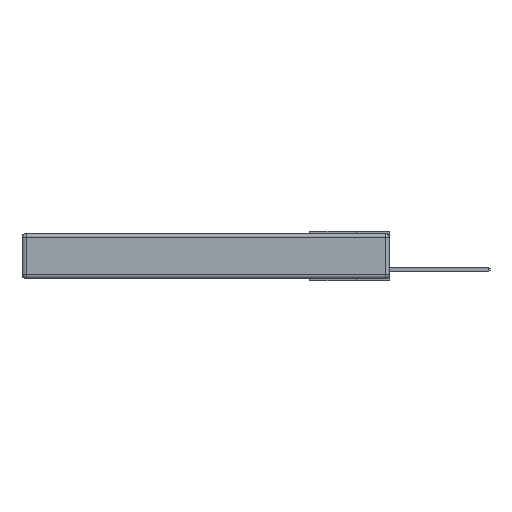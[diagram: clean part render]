
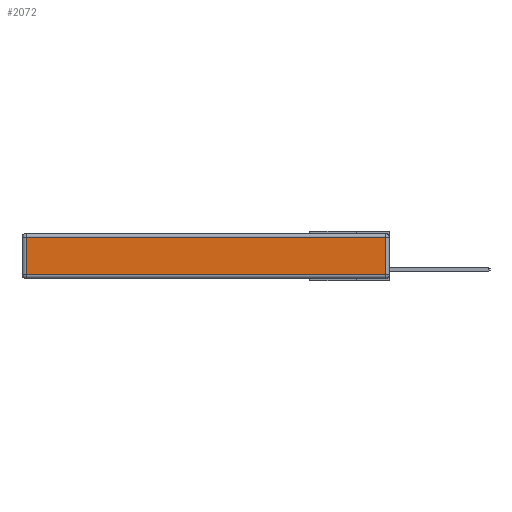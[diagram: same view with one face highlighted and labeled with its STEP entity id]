
A CAD part, left-side view. The second image highlights one B-rep face of the part: STEP entity #2072.
In plain terms, the highlighted planar face has unit normal (-1, 0, 0).
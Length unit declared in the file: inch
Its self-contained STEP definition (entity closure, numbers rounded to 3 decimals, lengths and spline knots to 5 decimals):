
#176 = CARTESIAN_POINT ( 'NONE',  ( 0., 0.03, -0.03 ) ) ;
#444 = VECTOR ( 'NONE', #2359, 39.37008 ) ;
#1381 = CARTESIAN_POINT ( 'NONE',  ( 0., 0.03, -0.313 ) ) ;
#2072 = ADVANCED_FACE ( 'NONE', ( #6727 ), #2088, .T. ) ;
#2088 = PLANE ( 'NONE',  #13191 ) ;
#2359 = DIRECTION ( 'NONE',  ( 0., 1., 0. ) ) ;
#3408 = VERTEX_POINT ( 'NONE', #4120 ) ;
#4120 = CARTESIAN_POINT ( 'NONE',  ( 0., 2.72, -0.313 ) ) ;
#4215 = DIRECTION ( 'NONE',  ( 0., 0., 1. ) ) ;
#4697 = LINE ( 'NONE', #11352, #8813 ) ;
#4736 = DIRECTION ( 'NONE',  ( 0., 0., 1. ) ) ;
#5076 = DIRECTION ( 'NONE',  ( 0., 0., -1. ) ) ;
#5177 = CARTESIAN_POINT ( 'NONE',  ( 0., 2.72, -0.03 ) ) ;
#5484 = CARTESIAN_POINT ( 'NONE',  ( 0., 0.03, -0.343 ) ) ;
#5848 = EDGE_CURVE ( 'NONE', #9457, #11286, #15091, .T. ) ;
#5866 = DIRECTION ( 'NONE',  ( 0., -1., 0. ) ) ;
#6336 = CARTESIAN_POINT ( 'NONE',  ( 0., 2.75, -0.03 ) ) ;
#6727 = FACE_OUTER_BOUND ( 'NONE', #15575, .T. ) ;
#7026 = ORIENTED_EDGE ( 'NONE', *, *, #15288, .T. ) ;
#8813 = VECTOR ( 'NONE', #5866, 39.37008 ) ;
#9131 = ORIENTED_EDGE ( 'NONE', *, *, #14897, .T. ) ;
#9163 = ORIENTED_EDGE ( 'NONE', *, *, #5848, .T. ) ;
#9457 = VERTEX_POINT ( 'NONE', #176 ) ;
#9525 = VERTEX_POINT ( 'NONE', #1381 ) ;
#10279 = CARTESIAN_POINT ( 'NONE',  ( 0., 0., -0.343 ) ) ;
#11286 = VERTEX_POINT ( 'NONE', #5177 ) ;
#11352 = CARTESIAN_POINT ( 'NONE',  ( 0., 0., -0.313 ) ) ;
#11611 = DIRECTION ( 'NONE',  ( -1., 0., 0. ) ) ;
#12475 = VECTOR ( 'NONE', #5076, 39.37008 ) ;
#12893 = VECTOR ( 'NONE', #4215, 39.37008 ) ;
#13191 = AXIS2_PLACEMENT_3D ( 'NONE', #10279, #11611, #4736 ) ;
#14405 = LINE ( 'NONE', #17434, #12475 ) ;
#14701 = EDGE_CURVE ( 'NONE', #11286, #3408, #14405, .T. ) ;
#14812 = ORIENTED_EDGE ( 'NONE', *, *, #14701, .T. ) ;
#14897 = EDGE_CURVE ( 'NONE', #3408, #9525, #4697, .T. ) ;
#15091 = LINE ( 'NONE', #6336, #444 ) ;
#15288 = EDGE_CURVE ( 'NONE', #9525, #9457, #16995, .T. ) ;
#15575 = EDGE_LOOP ( 'NONE', ( #9131, #7026, #9163, #14812 ) ) ;
#16995 = LINE ( 'NONE', #5484, #12893 ) ;
#17434 = CARTESIAN_POINT ( 'NONE',  ( 0., 2.72, -0.343 ) ) ;
